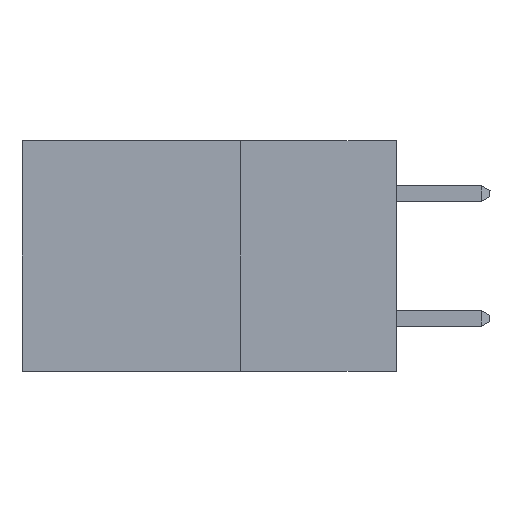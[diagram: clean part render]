
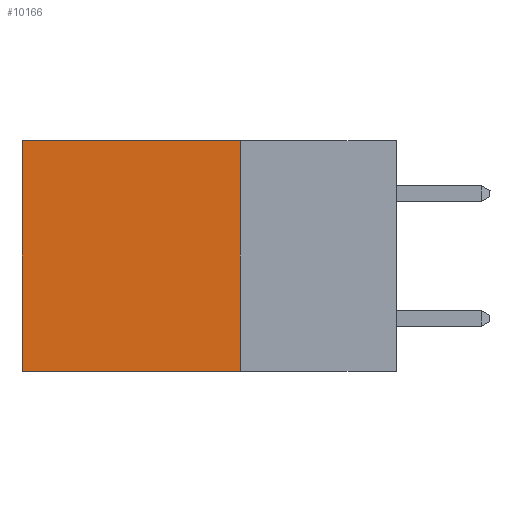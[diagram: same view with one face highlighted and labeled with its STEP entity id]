
A CAD part, left-side view. The second image highlights one B-rep face of the part: STEP entity #10166.
In plain terms, the highlighted planar face has unit normal (-1, 0, 0).
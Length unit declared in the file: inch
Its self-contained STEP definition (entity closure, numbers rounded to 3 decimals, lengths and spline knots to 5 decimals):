
#5 = ORIENTED_EDGE ( 'NONE', *, *, #9575, .T. ) ;
#605 = DIRECTION ( 'NONE',  ( 1., 0., 0. ) ) ;
#972 = CARTESIAN_POINT ( 'NONE',  ( 0.298, 0.25, -0.37 ) ) ;
#1223 = ORIENTED_EDGE ( 'NONE', *, *, #8667, .F. ) ;
#1237 = CARTESIAN_POINT ( 'NONE',  ( 0.298, 0.25, 0. ) ) ;
#1361 = CARTESIAN_POINT ( 'NONE',  ( 0.298, 0.25, 0. ) ) ;
#1530 = VECTOR ( 'NONE', #3870, 39.37008 ) ;
#1782 = ORIENTED_EDGE ( 'NONE', *, *, #8364, .F. ) ;
#2281 = VERTEX_POINT ( 'NONE', #8378 ) ;
#2500 = VERTEX_POINT ( 'NONE', #6591 ) ;
#2927 = ORIENTED_EDGE ( 'NONE', *, *, #9458, .T. ) ;
#3231 = LINE ( 'NONE', #1361, #7377 ) ;
#3870 = DIRECTION ( 'NONE',  ( 0., 0., -1. ) ) ;
#4251 = DIRECTION ( 'NONE',  ( 0., 1., 0. ) ) ;
#4279 = LINE ( 'NONE', #9879, #7004 ) ;
#4752 = CARTESIAN_POINT ( 'NONE',  ( 0.298, 0.6, 0. ) ) ;
#5371 = VERTEX_POINT ( 'NONE', #972 ) ;
#5628 = PLANE ( 'NONE',  #9781 ) ;
#6443 = DIRECTION ( 'NONE',  ( 0., 0., -1. ) ) ;
#6476 = CARTESIAN_POINT ( 'NONE',  ( 0.298, 0.6, -0.37 ) ) ;
#6591 = CARTESIAN_POINT ( 'NONE',  ( 0.298, 0.6, 0. ) ) ;
#6986 = VECTOR ( 'NONE', #7818, 39.37008 ) ;
#7004 = VECTOR ( 'NONE', #4251, 39.37008 ) ;
#7242 = LINE ( 'NONE', #1237, #6986 ) ;
#7377 = VECTOR ( 'NONE', #8744, 39.37008 ) ;
#7802 = VERTEX_POINT ( 'NONE', #6476 ) ;
#7818 = DIRECTION ( 'NONE',  ( 0., 1., 0. ) ) ;
#7875 = FACE_OUTER_BOUND ( 'NONE', #8151, .T. ) ;
#8151 = EDGE_LOOP ( 'NONE', ( #5, #1223, #1782, #2927 ) ) ;
#8364 = EDGE_CURVE ( 'NONE', #2281, #5371, #3231, .T. ) ;
#8378 = CARTESIAN_POINT ( 'NONE',  ( 0.298, 0.25, 0. ) ) ;
#8667 = EDGE_CURVE ( 'NONE', #5371, #7802, #4279, .T. ) ;
#8744 = DIRECTION ( 'NONE',  ( 0., 0., -1. ) ) ;
#9458 = EDGE_CURVE ( 'NONE', #2281, #2500, #7242, .T. ) ;
#9575 = EDGE_CURVE ( 'NONE', #2500, #7802, #10155, .T. ) ;
#9781 = AXIS2_PLACEMENT_3D ( 'NONE', #10345, #605, #6443 ) ;
#9879 = CARTESIAN_POINT ( 'NONE',  ( 0.298, 0.25, -0.37 ) ) ;
#10155 = LINE ( 'NONE', #4752, #1530 ) ;
#10166 = ADVANCED_FACE ( 'NONE', ( #7875 ), #5628, .F. ) ;
#10345 = CARTESIAN_POINT ( 'NONE',  ( 0.298, 0.25, 0. ) ) ;
